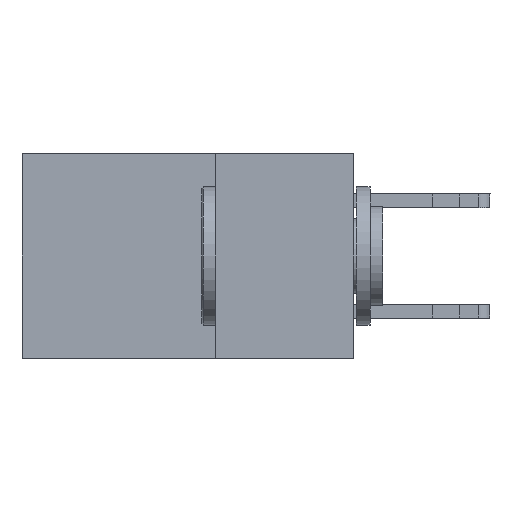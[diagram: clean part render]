
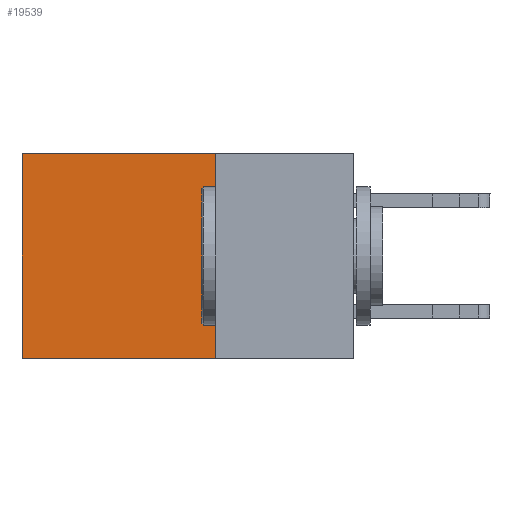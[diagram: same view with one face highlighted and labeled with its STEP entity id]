
A CAD part, left-side view. The second image highlights one B-rep face of the part: STEP entity #19539.
In plain terms, the highlighted planar face has unit normal (-1, 0, 0).
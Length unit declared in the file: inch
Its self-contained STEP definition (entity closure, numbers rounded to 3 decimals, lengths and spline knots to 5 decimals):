
#946 = PLANE ( 'NONE',  #20302 ) ;
#1137 = DIRECTION ( 'NONE',  ( 0., 0., -1. ) ) ;
#1571 = EDGE_CURVE ( 'NONE', #5935, #4410, #6881, .T. ) ;
#2132 = LINE ( 'NONE', #18613, #15063 ) ;
#3380 = EDGE_CURVE ( 'NONE', #6950, #10457, #11844, .T. ) ;
#3466 = LINE ( 'NONE', #10640, #13810 ) ;
#4410 = VERTEX_POINT ( 'NONE', #18948 ) ;
#4527 = FACE_OUTER_BOUND ( 'NONE', #7340, .T. ) ;
#5096 = DIRECTION ( 'NONE',  ( 0., 0., -1. ) ) ;
#5682 = CARTESIAN_POINT ( 'NONE',  ( 0.2875, 0.25, 0. ) ) ;
#5935 = VERTEX_POINT ( 'NONE', #16978 ) ;
#6881 = LINE ( 'NONE', #11792, #15299 ) ;
#6950 = VERTEX_POINT ( 'NONE', #5682 ) ;
#7340 = EDGE_LOOP ( 'NONE', ( #19950, #16575, #7821, #9078 ) ) ;
#7821 = ORIENTED_EDGE ( 'NONE', *, *, #3380, .F. ) ;
#9006 = CARTESIAN_POINT ( 'NONE',  ( 0.2875, 0.25, 0. ) ) ;
#9078 = ORIENTED_EDGE ( 'NONE', *, *, #23068, .T. ) ;
#9349 = VECTOR ( 'NONE', #15935, 39.37008 ) ;
#10457 = VERTEX_POINT ( 'NONE', #15215 ) ;
#10640 = CARTESIAN_POINT ( 'NONE',  ( 0.2875, 0.25, 0. ) ) ;
#11792 = CARTESIAN_POINT ( 'NONE',  ( 0.2875, 0.6, 0. ) ) ;
#11844 = LINE ( 'NONE', #9006, #9349 ) ;
#13810 = VECTOR ( 'NONE', #16065, 39.37008 ) ;
#14028 = EDGE_CURVE ( 'NONE', #10457, #4410, #2132, .T. ) ;
#15063 = VECTOR ( 'NONE', #16648, 39.37008 ) ;
#15215 = CARTESIAN_POINT ( 'NONE',  ( 0.2875, 0.25, -0.37 ) ) ;
#15299 = VECTOR ( 'NONE', #1137, 39.37008 ) ;
#15935 = DIRECTION ( 'NONE',  ( 0., 0., -1. ) ) ;
#16065 = DIRECTION ( 'NONE',  ( 0., 1., 0. ) ) ;
#16575 = ORIENTED_EDGE ( 'NONE', *, *, #14028, .F. ) ;
#16648 = DIRECTION ( 'NONE',  ( 0., 1., 0. ) ) ;
#16872 = CARTESIAN_POINT ( 'NONE',  ( 0.2875, 0.25, 0. ) ) ;
#16978 = CARTESIAN_POINT ( 'NONE',  ( 0.2875, 0.6, 0. ) ) ;
#18613 = CARTESIAN_POINT ( 'NONE',  ( 0.2875, 0.25, -0.37 ) ) ;
#18948 = CARTESIAN_POINT ( 'NONE',  ( 0.2875, 0.6, -0.37 ) ) ;
#19539 = ADVANCED_FACE ( 'NONE', ( #4527 ), #946, .F. ) ;
#19950 = ORIENTED_EDGE ( 'NONE', *, *, #1571, .T. ) ;
#20302 = AXIS2_PLACEMENT_3D ( 'NONE', #16872, #20855, #5096 ) ;
#20855 = DIRECTION ( 'NONE',  ( 1., 0., 0. ) ) ;
#23068 = EDGE_CURVE ( 'NONE', #6950, #5935, #3466, .T. ) ;
